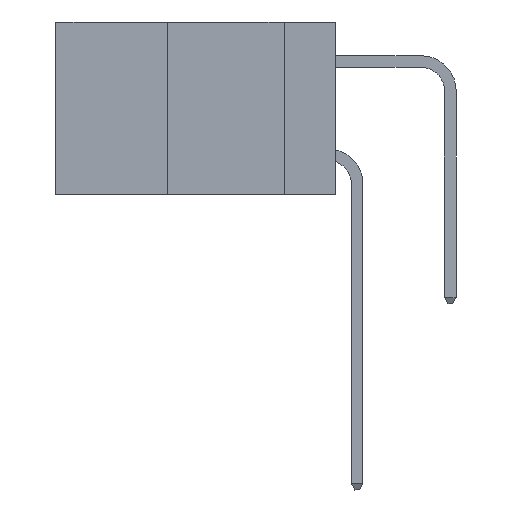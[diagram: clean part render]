
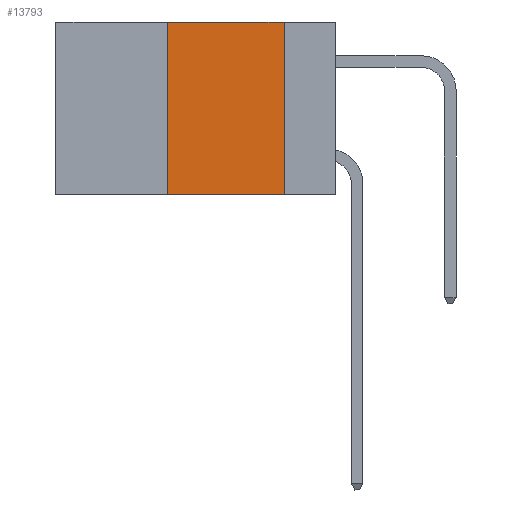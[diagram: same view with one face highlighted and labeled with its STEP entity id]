
A CAD part, left-side view. The second image highlights one B-rep face of the part: STEP entity #13793.
In plain terms, the highlighted planar face has unit normal (-1, 0, 0).
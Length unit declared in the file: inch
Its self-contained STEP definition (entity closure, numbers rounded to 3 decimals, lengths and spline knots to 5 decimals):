
#413 = CARTESIAN_POINT ( 'NONE',  ( 0., 0.36, 0. ) ) ;
#484 = VERTEX_POINT ( 'NONE', #17721 ) ;
#947 = LINE ( 'NONE', #413, #9126 ) ;
#2436 = DIRECTION ( 'NONE',  ( 0., 0., 1. ) ) ;
#2609 = DIRECTION ( 'NONE',  ( 1., 0., 0. ) ) ;
#2745 = EDGE_CURVE ( 'NONE', #15315, #484, #947, .T. ) ;
#4246 = ORIENTED_EDGE ( 'NONE', *, *, #21743, .F. ) ;
#4297 = CARTESIAN_POINT ( 'NONE',  ( 0., 0.6, 0. ) ) ;
#4737 = ORIENTED_EDGE ( 'NONE', *, *, #2745, .F. ) ;
#5059 = VERTEX_POINT ( 'NONE', #17235 ) ;
#5102 = LINE ( 'NONE', #24380, #14500 ) ;
#6149 = PLANE ( 'NONE',  #9732 ) ;
#6329 = DIRECTION ( 'NONE',  ( 0., 0., -1. ) ) ;
#7101 = DIRECTION ( 'NONE',  ( 0., -1., 0. ) ) ;
#8417 = CARTESIAN_POINT ( 'NONE',  ( 0., 0.36, -0.37 ) ) ;
#9126 = VECTOR ( 'NONE', #2436, 39.37008 ) ;
#9732 = AXIS2_PLACEMENT_3D ( 'NONE', #4297, #2609, #6329 ) ;
#10309 = EDGE_CURVE ( 'NONE', #15315, #5059, #5102, .T. ) ;
#10596 = FACE_OUTER_BOUND ( 'NONE', #18612, .T. ) ;
#13406 = ORIENTED_EDGE ( 'NONE', *, *, #10309, .T. ) ;
#13793 = ADVANCED_FACE ( 'NONE', ( #10596 ), #6149, .F. ) ;
#14500 = VECTOR ( 'NONE', #7101, 39.37008 ) ;
#15315 = VERTEX_POINT ( 'NONE', #8417 ) ;
#17235 = CARTESIAN_POINT ( 'NONE',  ( 0., 0.11, -0.37 ) ) ;
#17721 = CARTESIAN_POINT ( 'NONE',  ( 0., 0.36, 0. ) ) ;
#17885 = LINE ( 'NONE', #18115, #18188 ) ;
#18115 = CARTESIAN_POINT ( 'NONE',  ( 0., 0.11, 0. ) ) ;
#18188 = VECTOR ( 'NONE', #24085, 39.37008 ) ;
#18307 = EDGE_CURVE ( 'NONE', #484, #21865, #19269, .T. ) ;
#18612 = EDGE_LOOP ( 'NONE', ( #4246, #23011, #4737, #13406 ) ) ;
#18724 = CARTESIAN_POINT ( 'NONE',  ( 0., 0.6, 0. ) ) ;
#18943 = DIRECTION ( 'NONE',  ( 0., -1., 0. ) ) ;
#19269 = LINE ( 'NONE', #18724, #24423 ) ;
#21743 = EDGE_CURVE ( 'NONE', #21865, #5059, #17885, .T. ) ;
#21865 = VERTEX_POINT ( 'NONE', #22567 ) ;
#22567 = CARTESIAN_POINT ( 'NONE',  ( 0., 0.11, 0. ) ) ;
#23011 = ORIENTED_EDGE ( 'NONE', *, *, #18307, .F. ) ;
#24085 = DIRECTION ( 'NONE',  ( 0., 0., -1. ) ) ;
#24380 = CARTESIAN_POINT ( 'NONE',  ( 0., 0.6, -0.37 ) ) ;
#24423 = VECTOR ( 'NONE', #18943, 39.37008 ) ;
